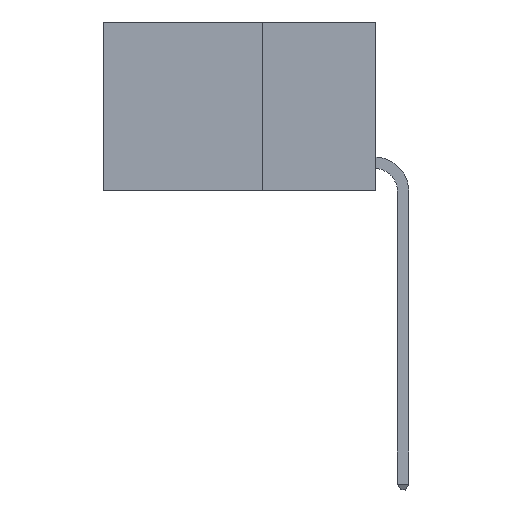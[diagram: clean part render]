
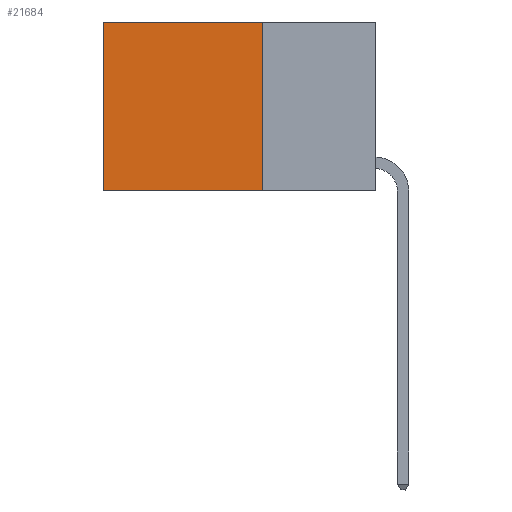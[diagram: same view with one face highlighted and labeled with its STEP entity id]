
A CAD part, left-side view. The second image highlights one B-rep face of the part: STEP entity #21684.
In plain terms, the highlighted planar face has unit normal (-1, 0, 0).
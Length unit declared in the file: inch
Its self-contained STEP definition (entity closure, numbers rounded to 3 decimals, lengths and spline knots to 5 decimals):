
#445 = CARTESIAN_POINT ( 'NONE',  ( 0.2625, 0.25, -0.37 ) ) ;
#658 = LINE ( 'NONE', #18808, #3184 ) ;
#662 = VERTEX_POINT ( 'NONE', #859 ) ;
#859 = CARTESIAN_POINT ( 'NONE',  ( 0.2625, 0.6, 0. ) ) ;
#1096 = ORIENTED_EDGE ( 'NONE', *, *, #10078, .T. ) ;
#1487 = VECTOR ( 'NONE', #15962, 39.37008 ) ;
#1623 = FACE_OUTER_BOUND ( 'NONE', #6957, .T. ) ;
#2541 = DIRECTION ( 'NONE',  ( 0., 1., 0. ) ) ;
#3059 = ORIENTED_EDGE ( 'NONE', *, *, #3664, .T. ) ;
#3184 = VECTOR ( 'NONE', #9785, 39.37008 ) ;
#3664 = EDGE_CURVE ( 'NONE', #5714, #662, #7845, .T. ) ;
#4342 = DIRECTION ( 'NONE',  ( 0., 0., -1. ) ) ;
#5102 = PLANE ( 'NONE',  #16016 ) ;
#5107 = VERTEX_POINT ( 'NONE', #12988 ) ;
#5714 = VERTEX_POINT ( 'NONE', #8981 ) ;
#5811 = VERTEX_POINT ( 'NONE', #445 ) ;
#6957 = EDGE_LOOP ( 'NONE', ( #1096, #18983, #19023, #3059 ) ) ;
#7845 = LINE ( 'NONE', #13753, #20495 ) ;
#8981 = CARTESIAN_POINT ( 'NONE',  ( 0.2625, 0.25, 0. ) ) ;
#9785 = DIRECTION ( 'NONE',  ( 0., 0., -1. ) ) ;
#10078 = EDGE_CURVE ( 'NONE', #662, #5107, #11806, .T. ) ;
#11018 = LINE ( 'NONE', #18349, #1487 ) ;
#11806 = LINE ( 'NONE', #15533, #23022 ) ;
#12099 = CARTESIAN_POINT ( 'NONE',  ( 0.2625, 0.25, 0. ) ) ;
#12213 = DIRECTION ( 'NONE',  ( 0., 0., -1. ) ) ;
#12988 = CARTESIAN_POINT ( 'NONE',  ( 0.2625, 0.6, -0.37 ) ) ;
#13753 = CARTESIAN_POINT ( 'NONE',  ( 0.2625, 0.25, 0. ) ) ;
#15533 = CARTESIAN_POINT ( 'NONE',  ( 0.2625, 0.6, 0. ) ) ;
#15962 = DIRECTION ( 'NONE',  ( 0., 1., 0. ) ) ;
#16016 = AXIS2_PLACEMENT_3D ( 'NONE', #12099, #23312, #12213 ) ;
#18349 = CARTESIAN_POINT ( 'NONE',  ( 0.2625, 0.25, -0.37 ) ) ;
#18808 = CARTESIAN_POINT ( 'NONE',  ( 0.2625, 0.25, 0. ) ) ;
#18983 = ORIENTED_EDGE ( 'NONE', *, *, #23356, .F. ) ;
#19023 = ORIENTED_EDGE ( 'NONE', *, *, #20093, .F. ) ;
#20093 = EDGE_CURVE ( 'NONE', #5714, #5811, #658, .T. ) ;
#20495 = VECTOR ( 'NONE', #2541, 39.37008 ) ;
#21684 = ADVANCED_FACE ( 'NONE', ( #1623 ), #5102, .F. ) ;
#23022 = VECTOR ( 'NONE', #4342, 39.37008 ) ;
#23312 = DIRECTION ( 'NONE',  ( 1., 0., 0. ) ) ;
#23356 = EDGE_CURVE ( 'NONE', #5811, #5107, #11018, .T. ) ;
